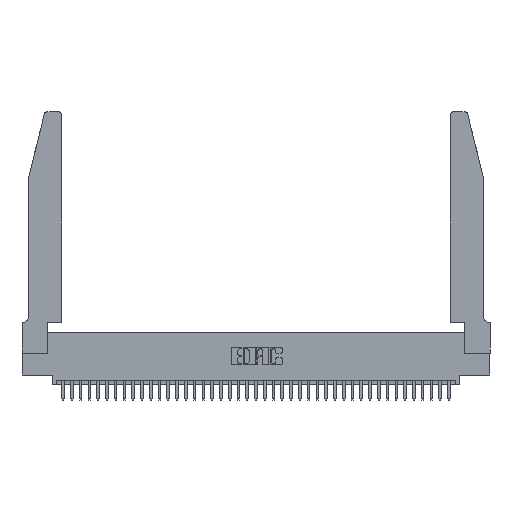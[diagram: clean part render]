
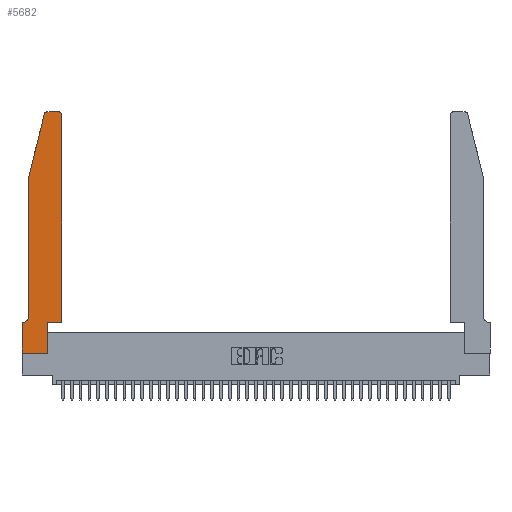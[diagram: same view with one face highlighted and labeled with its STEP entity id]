
A CAD part, top view. The second image highlights one B-rep face of the part: STEP entity #5682.
In plain terms, the highlighted planar face has unit normal (0, 0, 1).
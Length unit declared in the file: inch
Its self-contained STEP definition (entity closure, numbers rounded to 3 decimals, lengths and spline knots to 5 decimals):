
#99 = DIRECTION ( 'NONE',  ( 0., 1., 0. ) ) ;
#301 = ORIENTED_EDGE ( 'NONE', *, *, #35996, .T. ) ;
#595 = ORIENTED_EDGE ( 'NONE', *, *, #36012, .T. ) ;
#1458 = DIRECTION ( 'NONE',  ( 0., 0., 1. ) ) ;
#1531 = DIRECTION ( 'NONE',  ( 0., 0., 1. ) ) ;
#2512 = LINE ( 'NONE', #15238, #37642 ) ;
#2982 = LINE ( 'NONE', #8954, #34699 ) ;
#3513 = PLANE ( 'NONE',  #14229 ) ;
#3804 = VERTEX_POINT ( 'NONE', #14886 ) ;
#3832 = CARTESIAN_POINT ( 'NONE',  ( 0.2865, 0., 0.37 ) ) ;
#4436 = VERTEX_POINT ( 'NONE', #23721 ) ;
#4491 = ORIENTED_EDGE ( 'NONE', *, *, #17007, .T. ) ;
#4701 = DIRECTION ( 'NONE',  ( 0., 1., 0. ) ) ;
#4967 = LINE ( 'NONE', #30262, #9294 ) ;
#5682 = ADVANCED_FACE ( 'NONE', ( #14116 ), #3513, .T. ) ;
#6280 = DIRECTION ( 'NONE',  ( 0., -1., 0. ) ) ;
#6937 = CARTESIAN_POINT ( 'NONE',  ( 0., 0.35, 0.37 ) ) ;
#7074 = DIRECTION ( 'NONE',  ( -1., 0., 0. ) ) ;
#7335 = VECTOR ( 'NONE', #14227, 39.37008 ) ;
#7995 = ORIENTED_EDGE ( 'NONE', *, *, #17882, .T. ) ;
#8043 = VERTEX_POINT ( 'NONE', #25148 ) ;
#8263 = CARTESIAN_POINT ( 'NONE',  ( 0.4505, 0.35, 0.37 ) ) ;
#8844 = CIRCLE ( 'NONE', #39085, 0.03 ) ;
#8954 = CARTESIAN_POINT ( 'NONE',  ( 0.0755, 0.35, 0.37 ) ) ;
#9294 = VECTOR ( 'NONE', #7074, 39.37008 ) ;
#9329 = LINE ( 'NONE', #8263, #27626 ) ;
#9670 = VECTOR ( 'NONE', #4701, 39.37008 ) ;
#9679 = LINE ( 'NONE', #15038, #24181 ) ;
#10323 = VECTOR ( 'NONE', #99, 39.37008 ) ;
#10812 = EDGE_CURVE ( 'NONE', #8043, #26547, #25825, .T. ) ;
#13094 = VERTEX_POINT ( 'NONE', #24421 ) ;
#13296 = ORIENTED_EDGE ( 'NONE', *, *, #34686, .T. ) ;
#13798 = DIRECTION ( 'NONE',  ( 1., 0., 0. ) ) ;
#13955 = CARTESIAN_POINT ( 'NONE',  ( 0.0755, 2., 0.37 ) ) ;
#14002 = CARTESIAN_POINT ( 'NONE',  ( 0.284, 2.72, 0.37 ) ) ;
#14116 = FACE_OUTER_BOUND ( 'NONE', #17148, .T. ) ;
#14227 = DIRECTION ( 'NONE',  ( -0.239, -0.971, 0. ) ) ;
#14229 = AXIS2_PLACEMENT_3D ( 'NONE', #38376, #1458, #13798 ) ;
#14276 = CARTESIAN_POINT ( 'NONE',  ( 0.4205, 2.75, 0.37 ) ) ;
#14334 = VERTEX_POINT ( 'NONE', #30820 ) ;
#14870 = ORIENTED_EDGE ( 'NONE', *, *, #26332, .T. ) ;
#14886 = CARTESIAN_POINT ( 'NONE',  ( 0.0055, 0.35, 0.37 ) ) ;
#15038 = CARTESIAN_POINT ( 'NONE',  ( 0.0755, 2., 0.37 ) ) ;
#15238 = CARTESIAN_POINT ( 'NONE',  ( 0., 0., 0.37 ) ) ;
#15609 = CARTESIAN_POINT ( 'NONE',  ( 0.284, 2.75, 0.37 ) ) ;
#15986 = LINE ( 'NONE', #13955, #7335 ) ;
#17007 = EDGE_CURVE ( 'NONE', #35323, #4436, #15986, .T. ) ;
#17148 = EDGE_LOOP ( 'NONE', ( #20674, #13296, #4491, #24817, #20200, #301, #595, #21972, #7995, #14870, #19325, #22533 ) ) ;
#17309 = DIRECTION ( 'NONE',  ( 1., 0., 0. ) ) ;
#17521 = CARTESIAN_POINT ( 'NONE',  ( 0.4505, 2.72, 0.37 ) ) ;
#17825 = DIRECTION ( 'NONE',  ( 1., 0., 0. ) ) ;
#17882 = EDGE_CURVE ( 'NONE', #26547, #14334, #35191, .T. ) ;
#18402 = CIRCLE ( 'NONE', #23680, 0.03 ) ;
#18514 = VERTEX_POINT ( 'NONE', #35596 ) ;
#18558 = CARTESIAN_POINT ( 'NONE',  ( 0.4505, 0.35, 0.37 ) ) ;
#19261 = VERTEX_POINT ( 'NONE', #17521 ) ;
#19325 = ORIENTED_EDGE ( 'NONE', *, *, #39923, .T. ) ;
#20019 = CARTESIAN_POINT ( 'NONE',  ( 0.0055, 0.42, 0.37 ) ) ;
#20200 = ORIENTED_EDGE ( 'NONE', *, *, #33933, .T. ) ;
#20329 = EDGE_CURVE ( 'NONE', #32224, #37905, #4967, .T. ) ;
#20674 = ORIENTED_EDGE ( 'NONE', *, *, #20329, .T. ) ;
#21972 = ORIENTED_EDGE ( 'NONE', *, *, #10812, .T. ) ;
#22533 = ORIENTED_EDGE ( 'NONE', *, *, #27001, .T. ) ;
#23083 = DIRECTION ( 'NONE',  ( 1., 0., 0. ) ) ;
#23680 = AXIS2_PLACEMENT_3D ( 'NONE', #27375, #39657, #24579 ) ;
#23721 = CARTESIAN_POINT ( 'NONE',  ( 0.0755, 2., 0.37 ) ) ;
#24050 = DIRECTION ( 'NONE',  ( -1., 0., 0. ) ) ;
#24075 = VERTEX_POINT ( 'NONE', #6937 ) ;
#24181 = VECTOR ( 'NONE', #30248, 39.37008 ) ;
#24421 = CARTESIAN_POINT ( 'NONE',  ( 0.0755, 0.42, 0.37 ) ) ;
#24579 = DIRECTION ( 'NONE',  ( 1., 0., 0. ) ) ;
#24817 = ORIENTED_EDGE ( 'NONE', *, *, #27535, .T. ) ;
#25148 = CARTESIAN_POINT ( 'NONE',  ( 0., 0., 0.37 ) ) ;
#25715 = CIRCLE ( 'NONE', #34362, 0.07 ) ;
#25825 = LINE ( 'NONE', #35878, #39333 ) ;
#26332 = EDGE_CURVE ( 'NONE', #14334, #18514, #9329, .T. ) ;
#26547 = VERTEX_POINT ( 'NONE', #3832 ) ;
#27001 = EDGE_CURVE ( 'NONE', #19261, #32224, #18402, .T. ) ;
#27375 = CARTESIAN_POINT ( 'NONE',  ( 0.4205, 2.72, 0.37 ) ) ;
#27535 = EDGE_CURVE ( 'NONE', #4436, #13094, #9679, .T. ) ;
#27626 = VECTOR ( 'NONE', #17825, 39.37008 ) ;
#29409 = DIRECTION ( 'NONE',  ( -1., 0., 0. ) ) ;
#30248 = DIRECTION ( 'NONE',  ( 0., -1., 0. ) ) ;
#30262 = CARTESIAN_POINT ( 'NONE',  ( 0.2605, 2.75, 0.37 ) ) ;
#30529 = LINE ( 'NONE', #18558, #10323 ) ;
#30820 = CARTESIAN_POINT ( 'NONE',  ( 0.2865, 0.35, 0.37 ) ) ;
#32083 = DIRECTION ( 'NONE',  ( 0., 0., -1. ) ) ;
#32107 = CARTESIAN_POINT ( 'NONE',  ( 0.2865, 0.35, 0.37 ) ) ;
#32224 = VERTEX_POINT ( 'NONE', #14276 ) ;
#32915 = CARTESIAN_POINT ( 'NONE',  ( 0.25487, 2.72718, 0.37 ) ) ;
#33933 = EDGE_CURVE ( 'NONE', #13094, #3804, #25715, .T. ) ;
#34362 = AXIS2_PLACEMENT_3D ( 'NONE', #20019, #32083, #29409 ) ;
#34686 = EDGE_CURVE ( 'NONE', #37905, #35323, #8844, .T. ) ;
#34699 = VECTOR ( 'NONE', #24050, 39.37008 ) ;
#35191 = LINE ( 'NONE', #32107, #9670 ) ;
#35323 = VERTEX_POINT ( 'NONE', #32915 ) ;
#35596 = CARTESIAN_POINT ( 'NONE',  ( 0.4505, 0.35, 0.37 ) ) ;
#35878 = CARTESIAN_POINT ( 'NONE',  ( 0., 0., 0.37 ) ) ;
#35996 = EDGE_CURVE ( 'NONE', #3804, #24075, #2982, .T. ) ;
#36012 = EDGE_CURVE ( 'NONE', #24075, #8043, #2512, .T. ) ;
#37642 = VECTOR ( 'NONE', #6280, 39.37008 ) ;
#37905 = VERTEX_POINT ( 'NONE', #15609 ) ;
#38376 = CARTESIAN_POINT ( 'NONE',  ( 0., 0.35, 0.37 ) ) ;
#39085 = AXIS2_PLACEMENT_3D ( 'NONE', #14002, #1531, #23083 ) ;
#39333 = VECTOR ( 'NONE', #17309, 39.37008 ) ;
#39657 = DIRECTION ( 'NONE',  ( 0., 0., 1. ) ) ;
#39923 = EDGE_CURVE ( 'NONE', #18514, #19261, #30529, .T. ) ;
